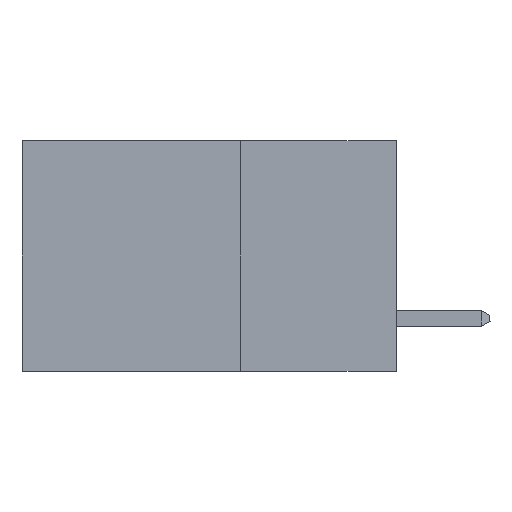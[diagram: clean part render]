
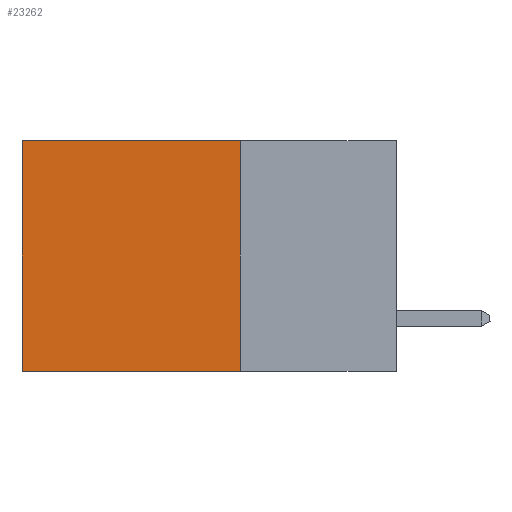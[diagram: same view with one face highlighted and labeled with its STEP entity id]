
A CAD part, left-side view. The second image highlights one B-rep face of the part: STEP entity #23262.
In plain terms, the highlighted planar face has unit normal (-1, 0, 0).
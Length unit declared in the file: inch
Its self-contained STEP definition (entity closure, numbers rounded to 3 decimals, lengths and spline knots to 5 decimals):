
#1196 = CARTESIAN_POINT ( 'NONE',  ( 0.298, 0.6, 0. ) ) ;
#1533 = ORIENTED_EDGE ( 'NONE', *, *, #6667, .T. ) ;
#1664 = ORIENTED_EDGE ( 'NONE', *, *, #7657, .T. ) ;
#6007 = CARTESIAN_POINT ( 'NONE',  ( 0.298, 0.25, -0.37 ) ) ;
#6072 = CARTESIAN_POINT ( 'NONE',  ( 0.298, 0.25, 0. ) ) ;
#6667 = EDGE_CURVE ( 'NONE', #21139, #6819, #19948, .T. ) ;
#6819 = VERTEX_POINT ( 'NONE', #1196 ) ;
#7657 = EDGE_CURVE ( 'NONE', #6819, #19896, #15231, .T. ) ;
#8323 = VERTEX_POINT ( 'NONE', #16800 ) ;
#8831 = CARTESIAN_POINT ( 'NONE',  ( 0.298, 0.25, 0. ) ) ;
#9168 = VECTOR ( 'NONE', #20568, 39.37008 ) ;
#10238 = CARTESIAN_POINT ( 'NONE',  ( 0.298, 0.6, 0. ) ) ;
#10929 = PLANE ( 'NONE',  #15401 ) ;
#11119 = DIRECTION ( 'NONE',  ( 0., 1., 0. ) ) ;
#11434 = EDGE_CURVE ( 'NONE', #8323, #19896, #14064, .T. ) ;
#12859 = EDGE_LOOP ( 'NONE', ( #1664, #18015, #18834, #1533 ) ) ;
#13041 = DIRECTION ( 'NONE',  ( 0., 0., -1. ) ) ;
#13295 = DIRECTION ( 'NONE',  ( 0., 0., -1. ) ) ;
#13726 = VECTOR ( 'NONE', #11119, 39.37008 ) ;
#14064 = LINE ( 'NONE', #6007, #9168 ) ;
#14577 = VECTOR ( 'NONE', #24749, 39.37008 ) ;
#14992 = VECTOR ( 'NONE', #13295, 39.37008 ) ;
#15231 = LINE ( 'NONE', #10238, #14577 ) ;
#15401 = AXIS2_PLACEMENT_3D ( 'NONE', #8831, #25353, #13041 ) ;
#16800 = CARTESIAN_POINT ( 'NONE',  ( 0.298, 0.25, -0.37 ) ) ;
#17254 = CARTESIAN_POINT ( 'NONE',  ( 0.298, 0.25, 0. ) ) ;
#18015 = ORIENTED_EDGE ( 'NONE', *, *, #11434, .F. ) ;
#18834 = ORIENTED_EDGE ( 'NONE', *, *, #24497, .F. ) ;
#19510 = CARTESIAN_POINT ( 'NONE',  ( 0.298, 0.25, 0. ) ) ;
#19896 = VERTEX_POINT ( 'NONE', #21294 ) ;
#19948 = LINE ( 'NONE', #17254, #13726 ) ;
#20554 = LINE ( 'NONE', #19510, #14992 ) ;
#20568 = DIRECTION ( 'NONE',  ( 0., 1., 0. ) ) ;
#21139 = VERTEX_POINT ( 'NONE', #6072 ) ;
#21294 = CARTESIAN_POINT ( 'NONE',  ( 0.298, 0.6, -0.37 ) ) ;
#22200 = FACE_OUTER_BOUND ( 'NONE', #12859, .T. ) ;
#23262 = ADVANCED_FACE ( 'NONE', ( #22200 ), #10929, .F. ) ;
#24497 = EDGE_CURVE ( 'NONE', #21139, #8323, #20554, .T. ) ;
#24749 = DIRECTION ( 'NONE',  ( 0., 0., -1. ) ) ;
#25353 = DIRECTION ( 'NONE',  ( 1., 0., 0. ) ) ;
